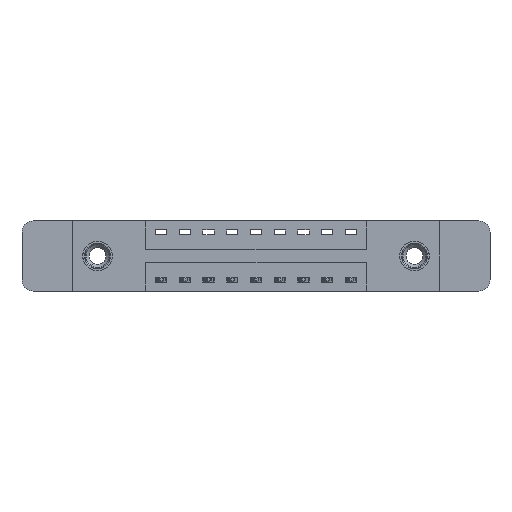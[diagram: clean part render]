
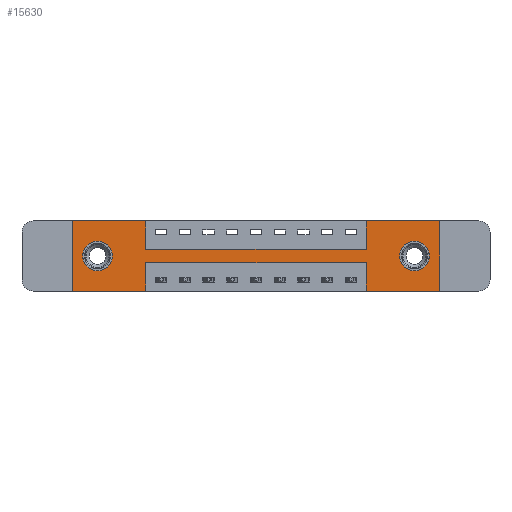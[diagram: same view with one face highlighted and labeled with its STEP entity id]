
A CAD part, front view. The second image highlights one B-rep face of the part: STEP entity #15630.
In plain terms, the highlighted planar face has unit normal (0, -1, 0).
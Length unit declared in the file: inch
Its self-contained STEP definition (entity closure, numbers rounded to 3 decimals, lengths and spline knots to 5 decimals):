
#289 = ORIENTED_EDGE ( 'NONE', *, *, #4826, .F. ) ;
#301 = DIRECTION ( 'NONE',  ( 0., 1., 0. ) ) ;
#309 = CARTESIAN_POINT ( 'NONE',  ( 0., 0., 0. ) ) ;
#463 = CARTESIAN_POINT ( 'NONE',  ( 1.8025, 0., -0.185 ) ) ;
#502 = LINE ( 'NONE', #13749, #9728 ) ;
#535 = CARTESIAN_POINT ( 'NONE',  ( 0.3875, 0., -0.22 ) ) ;
#564 = VERTEX_POINT ( 'NONE', #12517 ) ;
#574 = DIRECTION ( 'NONE',  ( 0., 0., 1. ) ) ;
#608 = CARTESIAN_POINT ( 'NONE',  ( 0., 0., 0. ) ) ;
#736 = ORIENTED_EDGE ( 'NONE', *, *, #3321, .T. ) ;
#757 = EDGE_CURVE ( 'NONE', #1182, #12764, #14900, .T. ) ;
#793 = VERTEX_POINT ( 'NONE', #535 ) ;
#824 = ORIENTED_EDGE ( 'NONE', *, *, #9903, .T. ) ;
#1150 = VERTEX_POINT ( 'NONE', #3012 ) ;
#1156 = CARTESIAN_POINT ( 'NONE',  ( 0.3875, 0., 0. ) ) ;
#1182 = VERTEX_POINT ( 'NONE', #13917 ) ;
#1214 = ORIENTED_EDGE ( 'NONE', *, *, #7080, .F. ) ;
#1396 = CARTESIAN_POINT ( 'NONE',  ( 0., 0., 0. ) ) ;
#1563 = ORIENTED_EDGE ( 'NONE', *, *, #6338, .F. ) ;
#1590 = DIRECTION ( 'NONE',  ( 0., 0., -1. ) ) ;
#1698 = VERTEX_POINT ( 'NONE', #1156 ) ;
#1769 = DIRECTION ( 'NONE',  ( -1., 0., 0. ) ) ;
#1861 = VERTEX_POINT ( 'NONE', #9531 ) ;
#1974 = AXIS2_PLACEMENT_3D ( 'NONE', #7955, #3032, #11477 ) ;
#2016 = DIRECTION ( 'NONE',  ( 0., 0., -1. ) ) ;
#2085 = FACE_BOUND ( 'NONE', #7149, .T. ) ;
#2386 = PLANE ( 'NONE',  #6840 ) ;
#2433 = EDGE_LOOP ( 'NONE', ( #11451, #11686 ) ) ;
#2462 = LINE ( 'NONE', #4115, #10355 ) ;
#2521 = ORIENTED_EDGE ( 'NONE', *, *, #4675, .F. ) ;
#2632 = DIRECTION ( 'NONE',  ( 0., 0., 1. ) ) ;
#2651 = DIRECTION ( 'NONE',  ( 0., 0., -1. ) ) ;
#2931 = DIRECTION ( 'NONE',  ( 0., 0., -1. ) ) ;
#3012 = CARTESIAN_POINT ( 'NONE',  ( 0.1325, 0., -0.263 ) ) ;
#3032 = DIRECTION ( 'NONE',  ( 0., 1., 0. ) ) ;
#3071 = AXIS2_PLACEMENT_3D ( 'NONE', #6775, #5502, #4457 ) ;
#3224 = CARTESIAN_POINT ( 'NONE',  ( 1.935, 0., 0. ) ) ;
#3321 = EDGE_CURVE ( 'NONE', #1150, #14705, #10685, .T. ) ;
#3336 = LINE ( 'NONE', #608, #11241 ) ;
#3643 = EDGE_LOOP ( 'NONE', ( #9891, #7881, #289, #11826, #11049, #9581, #11859, #3705, #1563, #2521, #5762, #1214 ) ) ;
#3646 = EDGE_CURVE ( 'NONE', #7035, #4425, #6522, .T. ) ;
#3703 = CARTESIAN_POINT ( 'NONE',  ( 1.8025, 0., -0.107 ) ) ;
#3705 = ORIENTED_EDGE ( 'NONE', *, *, #11526, .F. ) ;
#3805 = LINE ( 'NONE', #13534, #10782 ) ;
#4115 = CARTESIAN_POINT ( 'NONE',  ( 0.3875, 0., -0.22 ) ) ;
#4195 = EDGE_CURVE ( 'NONE', #793, #1861, #12916, .T. ) ;
#4211 = CARTESIAN_POINT ( 'NONE',  ( 1.935, 0., -0.37 ) ) ;
#4281 = LINE ( 'NONE', #11763, #7924 ) ;
#4425 = VERTEX_POINT ( 'NONE', #7477 ) ;
#4457 = DIRECTION ( 'NONE',  ( 0., 0., 1. ) ) ;
#4476 = CARTESIAN_POINT ( 'NONE',  ( 0.3875, 0., -0.37 ) ) ;
#4529 = DIRECTION ( 'NONE',  ( 0., 0., 1. ) ) ;
#4675 = EDGE_CURVE ( 'NONE', #13859, #1698, #3336, .T. ) ;
#4765 = FACE_OUTER_BOUND ( 'NONE', #3643, .T. ) ;
#4826 = EDGE_CURVE ( 'NONE', #4425, #5661, #4917, .T. ) ;
#4891 = EDGE_CURVE ( 'NONE', #14732, #7035, #4281, .T. ) ;
#4917 = LINE ( 'NONE', #9761, #6674 ) ;
#4998 = DIRECTION ( 'NONE',  ( -1., 0., 0. ) ) ;
#5050 = LINE ( 'NONE', #1396, #10534 ) ;
#5427 = DIRECTION ( 'NONE',  ( 1., 0., 0. ) ) ;
#5502 = DIRECTION ( 'NONE',  ( 0., 1., 0. ) ) ;
#5661 = VERTEX_POINT ( 'NONE', #14870 ) ;
#5760 = VERTEX_POINT ( 'NONE', #12237 ) ;
#5762 = ORIENTED_EDGE ( 'NONE', *, *, #9673, .F. ) ;
#5822 = DIRECTION ( 'NONE',  ( 0., -1., 0. ) ) ;
#5933 = VERTEX_POINT ( 'NONE', #12579 ) ;
#6019 = VECTOR ( 'NONE', #12958, 39.37008 ) ;
#6053 = VECTOR ( 'NONE', #574, 39.37008 ) ;
#6162 = VECTOR ( 'NONE', #2016, 39.37008 ) ;
#6338 = EDGE_CURVE ( 'NONE', #1698, #5760, #502, .T. ) ;
#6516 = AXIS2_PLACEMENT_3D ( 'NONE', #463, #301, #2651 ) ;
#6522 = LINE ( 'NONE', #7453, #9671 ) ;
#6674 = VECTOR ( 'NONE', #13436, 39.37008 ) ;
#6775 = CARTESIAN_POINT ( 'NONE',  ( 0.1325, 0., -0.185 ) ) ;
#6840 = AXIS2_PLACEMENT_3D ( 'NONE', #12984, #5822, #9612 ) ;
#7035 = VERTEX_POINT ( 'NONE', #4211 ) ;
#7080 = EDGE_CURVE ( 'NONE', #1861, #564, #11227, .T. ) ;
#7129 = CARTESIAN_POINT ( 'NONE',  ( 0.3875, 0., -0.15 ) ) ;
#7149 = EDGE_LOOP ( 'NONE', ( #824, #736 ) ) ;
#7453 = CARTESIAN_POINT ( 'NONE',  ( 0., 0., -0.37 ) ) ;
#7475 = CARTESIAN_POINT ( 'NONE',  ( 0., 0., -0.37 ) ) ;
#7477 = CARTESIAN_POINT ( 'NONE',  ( 1.5475, 0., -0.37 ) ) ;
#7731 = VECTOR ( 'NONE', #1769, 39.37008 ) ;
#7881 = ORIENTED_EDGE ( 'NONE', *, *, #12482, .F. ) ;
#7924 = VECTOR ( 'NONE', #2931, 39.37008 ) ;
#7955 = CARTESIAN_POINT ( 'NONE',  ( 1.8025, 0., -0.185 ) ) ;
#8172 = DIRECTION ( 'NONE',  ( 0., 1., 0. ) ) ;
#8699 = DIRECTION ( 'NONE',  ( 1., 0., 0. ) ) ;
#8952 = CARTESIAN_POINT ( 'NONE',  ( 1.5475, 0., 0. ) ) ;
#9224 = FACE_BOUND ( 'NONE', #2433, .T. ) ;
#9312 = EDGE_CURVE ( 'NONE', #13166, #14732, #5050, .T. ) ;
#9531 = CARTESIAN_POINT ( 'NONE',  ( 0.3875, 0., -0.37 ) ) ;
#9581 = ORIENTED_EDGE ( 'NONE', *, *, #9312, .F. ) ;
#9612 = DIRECTION ( 'NONE',  ( 0., 0., -1. ) ) ;
#9671 = VECTOR ( 'NONE', #4998, 39.37008 ) ;
#9673 = EDGE_CURVE ( 'NONE', #564, #13859, #3805, .T. ) ;
#9728 = VECTOR ( 'NONE', #1590, 39.37008 ) ;
#9761 = CARTESIAN_POINT ( 'NONE',  ( 1.5475, 0., -0.37 ) ) ;
#9891 = ORIENTED_EDGE ( 'NONE', *, *, #4195, .F. ) ;
#9903 = EDGE_CURVE ( 'NONE', #14705, #1150, #11057, .T. ) ;
#10301 = AXIS2_PLACEMENT_3D ( 'NONE', #15395, #8172, #4529 ) ;
#10355 = VECTOR ( 'NONE', #12802, 39.37008 ) ;
#10430 = EDGE_CURVE ( 'NONE', #12764, #1182, #13878, .T. ) ;
#10534 = VECTOR ( 'NONE', #8699, 39.37008 ) ;
#10685 = CIRCLE ( 'NONE', #3071, 0.078 ) ;
#10782 = VECTOR ( 'NONE', #2632, 39.37008 ) ;
#11049 = ORIENTED_EDGE ( 'NONE', *, *, #4891, .F. ) ;
#11057 = CIRCLE ( 'NONE', #10301, 0.078 ) ;
#11227 = LINE ( 'NONE', #7475, #7731 ) ;
#11241 = VECTOR ( 'NONE', #5427, 39.37008 ) ;
#11434 = LINE ( 'NONE', #8952, #6053 ) ;
#11451 = ORIENTED_EDGE ( 'NONE', *, *, #10430, .T. ) ;
#11477 = DIRECTION ( 'NONE',  ( 0., 0., -1. ) ) ;
#11517 = CARTESIAN_POINT ( 'NONE',  ( 0.1325, 0., -0.107 ) ) ;
#11526 = EDGE_CURVE ( 'NONE', #5760, #5933, #11837, .T. ) ;
#11686 = ORIENTED_EDGE ( 'NONE', *, *, #757, .T. ) ;
#11763 = CARTESIAN_POINT ( 'NONE',  ( 1.935, 0., 0. ) ) ;
#11826 = ORIENTED_EDGE ( 'NONE', *, *, #3646, .F. ) ;
#11837 = LINE ( 'NONE', #7129, #6019 ) ;
#11859 = ORIENTED_EDGE ( 'NONE', *, *, #12888, .F. ) ;
#12237 = CARTESIAN_POINT ( 'NONE',  ( 0.3875, 0., -0.15 ) ) ;
#12482 = EDGE_CURVE ( 'NONE', #5661, #793, #2462, .T. ) ;
#12517 = CARTESIAN_POINT ( 'NONE',  ( 0., 0., -0.37 ) ) ;
#12579 = CARTESIAN_POINT ( 'NONE',  ( 1.5475, 0., -0.15 ) ) ;
#12764 = VERTEX_POINT ( 'NONE', #3703 ) ;
#12802 = DIRECTION ( 'NONE',  ( -1., 0., 0. ) ) ;
#12888 = EDGE_CURVE ( 'NONE', #5933, #13166, #11434, .T. ) ;
#12916 = LINE ( 'NONE', #4476, #6162 ) ;
#12958 = DIRECTION ( 'NONE',  ( 1., 0., 0. ) ) ;
#12984 = CARTESIAN_POINT ( 'NONE',  ( 0., 0., -0.37 ) ) ;
#13166 = VERTEX_POINT ( 'NONE', #14015 ) ;
#13436 = DIRECTION ( 'NONE',  ( 0., 0., 1. ) ) ;
#13534 = CARTESIAN_POINT ( 'NONE',  ( 0., 0., 0. ) ) ;
#13749 = CARTESIAN_POINT ( 'NONE',  ( 0.3875, 0., 0. ) ) ;
#13859 = VERTEX_POINT ( 'NONE', #309 ) ;
#13878 = CIRCLE ( 'NONE', #6516, 0.078 ) ;
#13917 = CARTESIAN_POINT ( 'NONE',  ( 1.8025, 0., -0.263 ) ) ;
#14015 = CARTESIAN_POINT ( 'NONE',  ( 1.5475, 0., 0. ) ) ;
#14705 = VERTEX_POINT ( 'NONE', #11517 ) ;
#14732 = VERTEX_POINT ( 'NONE', #3224 ) ;
#14870 = CARTESIAN_POINT ( 'NONE',  ( 1.5475, 0., -0.22 ) ) ;
#14900 = CIRCLE ( 'NONE', #1974, 0.078 ) ;
#15395 = CARTESIAN_POINT ( 'NONE',  ( 0.1325, 0., -0.185 ) ) ;
#15630 = ADVANCED_FACE ( 'NONE', ( #9224, #2085, #4765 ), #2386, .T. ) ;
